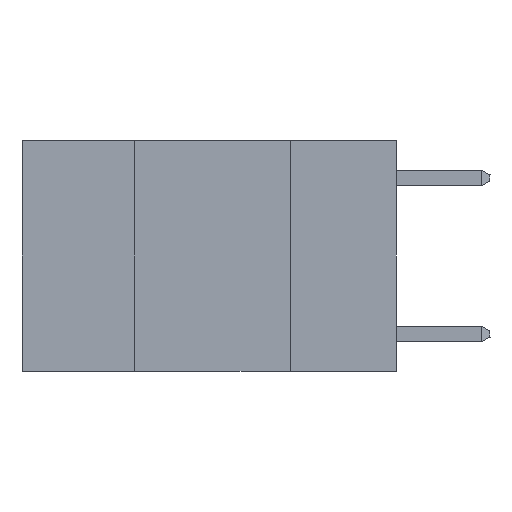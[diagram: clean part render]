
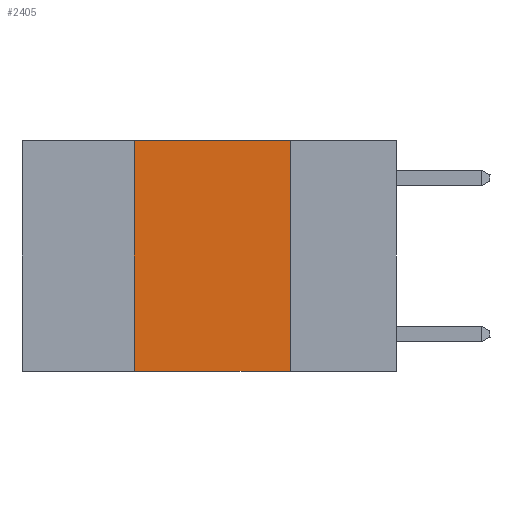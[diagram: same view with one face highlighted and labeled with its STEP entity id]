
A CAD part, left-side view. The second image highlights one B-rep face of the part: STEP entity #2405.
In plain terms, the highlighted planar face has unit normal (-1, 0, 0).
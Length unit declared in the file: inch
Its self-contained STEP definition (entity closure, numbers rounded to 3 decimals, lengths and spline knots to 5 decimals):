
#247 = ORIENTED_EDGE ( 'NONE', *, *, #12099, .T. ) ;
#362 = LINE ( 'NONE', #10229, #12644 ) ;
#426 = DIRECTION ( 'NONE',  ( 0., -1., 0. ) ) ;
#464 = VERTEX_POINT ( 'NONE', #8875 ) ;
#641 = VECTOR ( 'NONE', #12663, 39.37008 ) ;
#1069 = VERTEX_POINT ( 'NONE', #2658 ) ;
#1201 = EDGE_CURVE ( 'NONE', #9613, #464, #4027, .T. ) ;
#1928 = ORIENTED_EDGE ( 'NONE', *, *, #7485, .F. ) ;
#2405 = ADVANCED_FACE ( 'NONE', ( #10220 ), #8347, .F. ) ;
#2424 = AXIS2_PLACEMENT_3D ( 'NONE', #7383, #5198, #11018 ) ;
#2658 = CARTESIAN_POINT ( 'NONE',  ( 0., 0.17, -0.37 ) ) ;
#2714 = LINE ( 'NONE', #11510, #8279 ) ;
#4027 = LINE ( 'NONE', #7912, #5878 ) ;
#4252 = ORIENTED_EDGE ( 'NONE', *, *, #11415, .F. ) ;
#4850 = LINE ( 'NONE', #10445, #641 ) ;
#5198 = DIRECTION ( 'NONE',  ( 1., 0., 0. ) ) ;
#5878 = VECTOR ( 'NONE', #7844, 39.37008 ) ;
#6646 = DIRECTION ( 'NONE',  ( 0., 0., -1. ) ) ;
#6722 = ORIENTED_EDGE ( 'NONE', *, *, #1201, .F. ) ;
#7077 = VERTEX_POINT ( 'NONE', #7716 ) ;
#7383 = CARTESIAN_POINT ( 'NONE',  ( 0., 0.6, 0. ) ) ;
#7485 = EDGE_CURVE ( 'NONE', #464, #1069, #2714, .T. ) ;
#7716 = CARTESIAN_POINT ( 'NONE',  ( 0., 0.42, -0.37 ) ) ;
#7844 = DIRECTION ( 'NONE',  ( 0., -1., 0. ) ) ;
#7912 = CARTESIAN_POINT ( 'NONE',  ( 0., 0.6, 0. ) ) ;
#8279 = VECTOR ( 'NONE', #6646, 39.37008 ) ;
#8290 = CARTESIAN_POINT ( 'NONE',  ( 0., 0.42, 0. ) ) ;
#8347 = PLANE ( 'NONE',  #2424 ) ;
#8875 = CARTESIAN_POINT ( 'NONE',  ( 0., 0.17, 0. ) ) ;
#9613 = VERTEX_POINT ( 'NONE', #8290 ) ;
#10220 = FACE_OUTER_BOUND ( 'NONE', #11180, .T. ) ;
#10229 = CARTESIAN_POINT ( 'NONE',  ( 0., 0.6, -0.37 ) ) ;
#10445 = CARTESIAN_POINT ( 'NONE',  ( 0., 0.42, 0. ) ) ;
#11018 = DIRECTION ( 'NONE',  ( 0., 0., -1. ) ) ;
#11180 = EDGE_LOOP ( 'NONE', ( #1928, #6722, #4252, #247 ) ) ;
#11415 = EDGE_CURVE ( 'NONE', #7077, #9613, #4850, .T. ) ;
#11510 = CARTESIAN_POINT ( 'NONE',  ( 0., 0.17, 0. ) ) ;
#12099 = EDGE_CURVE ( 'NONE', #7077, #1069, #362, .T. ) ;
#12644 = VECTOR ( 'NONE', #426, 39.37008 ) ;
#12663 = DIRECTION ( 'NONE',  ( 0., 0., 1. ) ) ;
